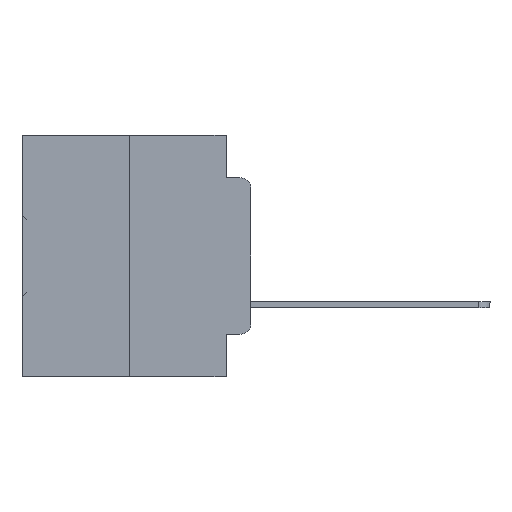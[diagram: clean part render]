
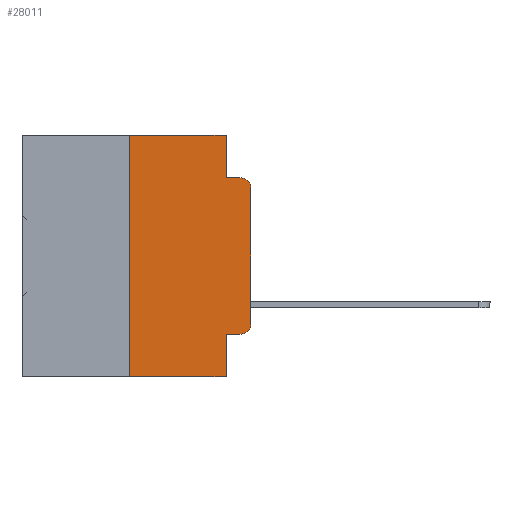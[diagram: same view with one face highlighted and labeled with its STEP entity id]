
A CAD part, left-side view. The second image highlights one B-rep face of the part: STEP entity #28011.
In plain terms, the highlighted planar face has unit normal (-1, 0, 0).
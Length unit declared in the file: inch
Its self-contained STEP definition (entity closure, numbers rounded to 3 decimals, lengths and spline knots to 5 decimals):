
#132 = VECTOR ( 'NONE', #17578, 39.37008 ) ;
#2353 = VERTEX_POINT ( 'NONE', #35481 ) ;
#2831 = DIRECTION ( 'NONE',  ( 0., 0., -1. ) ) ;
#4867 = VERTEX_POINT ( 'NONE', #15763 ) ;
#5420 = ORIENTED_EDGE ( 'NONE', *, *, #31383, .T. ) ;
#5552 = EDGE_CURVE ( 'NONE', #30710, #17020, #28559, .T. ) ;
#5701 = EDGE_CURVE ( 'NONE', #6579, #4867, #35004, .T. ) ;
#6166 = VECTOR ( 'NONE', #27151, 39.37008 ) ;
#6307 = VERTEX_POINT ( 'NONE', #22232 ) ;
#6451 = VECTOR ( 'NONE', #31825, 39.37008 ) ;
#6579 = VERTEX_POINT ( 'NONE', #26441 ) ;
#6955 = CARTESIAN_POINT ( 'NONE',  ( 0., 0.051, 0. ) ) ;
#7369 = ORIENTED_EDGE ( 'NONE', *, *, #24601, .F. ) ;
#7588 = VECTOR ( 'NONE', #8814, 39.37008 ) ;
#7615 = VERTEX_POINT ( 'NONE', #15172 ) ;
#8107 = CIRCLE ( 'NONE', #23387, 0.02 ) ;
#8814 = DIRECTION ( 'NONE',  ( 0., 0., 1. ) ) ;
#8893 = ORIENTED_EDGE ( 'NONE', *, *, #24710, .T. ) ;
#9020 = DIRECTION ( 'NONE',  ( 0., -1., 0. ) ) ;
#9354 = LINE ( 'NONE', #6955, #6451 ) ;
#9924 = ORIENTED_EDGE ( 'NONE', *, *, #27396, .F. ) ;
#10054 = VERTEX_POINT ( 'NONE', #34585 ) ;
#11813 = ORIENTED_EDGE ( 'NONE', *, *, #5701, .T. ) ;
#12061 = LINE ( 'NONE', #31401, #132 ) ;
#12445 = EDGE_CURVE ( 'NONE', #6579, #7615, #9354, .T. ) ;
#15172 = CARTESIAN_POINT ( 'NONE',  ( 0., 0.051, -0.5 ) ) ;
#15763 = CARTESIAN_POINT ( 'NONE',  ( 0., 0.02, -0.4115 ) ) ;
#16089 = LINE ( 'NONE', #27339, #6166 ) ;
#16677 = VERTEX_POINT ( 'NONE', #23759 ) ;
#16905 = CARTESIAN_POINT ( 'NONE',  ( 0., 0., -0.3915 ) ) ;
#16954 = DIRECTION ( 'NONE',  ( 0., 0., -1. ) ) ;
#17020 = VERTEX_POINT ( 'NONE', #25204 ) ;
#17578 = DIRECTION ( 'NONE',  ( 0., 0., -1. ) ) ;
#17596 = CARTESIAN_POINT ( 'NONE',  ( 0., 0.473, 0. ) ) ;
#17858 = DIRECTION ( 'NONE',  ( 1., 0., 0. ) ) ;
#18437 = ORIENTED_EDGE ( 'NONE', *, *, #36356, .F. ) ;
#18599 = ORIENTED_EDGE ( 'NONE', *, *, #12445, .F. ) ;
#19317 = EDGE_LOOP ( 'NONE', ( #5420, #32212, #31492, #18437, #9924, #7369, #24969, #18599, #11813, #8893 ) ) ;
#19327 = AXIS2_PLACEMENT_3D ( 'NONE', #20994, #17858, #29653 ) ;
#19458 = VERTEX_POINT ( 'NONE', #16905 ) ;
#20444 = VECTOR ( 'NONE', #31789, 39.37008 ) ;
#20994 = CARTESIAN_POINT ( 'NONE',  ( 0., 0.473, 0. ) ) ;
#22232 = CARTESIAN_POINT ( 'NONE',  ( 0., 0., -0.1085 ) ) ;
#23070 = DIRECTION ( 'NONE',  ( -1., 0., 0. ) ) ;
#23387 = AXIS2_PLACEMENT_3D ( 'NONE', #28196, #31681, #16954 ) ;
#23759 = CARTESIAN_POINT ( 'NONE',  ( 0., 0.051, 0. ) ) ;
#24179 = LINE ( 'NONE', #35405, #32360 ) ;
#24601 = EDGE_CURVE ( 'NONE', #2353, #10054, #16089, .T. ) ;
#24710 = EDGE_CURVE ( 'NONE', #4867, #19458, #26739, .T. ) ;
#24969 = ORIENTED_EDGE ( 'NONE', *, *, #34084, .T. ) ;
#24986 = VECTOR ( 'NONE', #9020, 39.37008 ) ;
#25204 = CARTESIAN_POINT ( 'NONE',  ( 0., 0.02, -0.0885 ) ) ;
#26441 = CARTESIAN_POINT ( 'NONE',  ( 0., 0.051, -0.4115 ) ) ;
#26739 = CIRCLE ( 'NONE', #29680, 0.02 ) ;
#27151 = DIRECTION ( 'NONE',  ( 0., 0., 1. ) ) ;
#27339 = CARTESIAN_POINT ( 'NONE',  ( 0., 0.25, 0. ) ) ;
#27396 = EDGE_CURVE ( 'NONE', #10054, #16677, #34922, .T. ) ;
#27898 = EDGE_CURVE ( 'NONE', #6307, #17020, #8107, .T. ) ;
#28011 = ADVANCED_FACE ( 'NONE', ( #29118 ), #35173, .F. ) ;
#28196 = CARTESIAN_POINT ( 'NONE',  ( 0., 0.02, -0.1085 ) ) ;
#28538 = LINE ( 'NONE', #34056, #7588 ) ;
#28559 = LINE ( 'NONE', #34450, #24986 ) ;
#29118 = FACE_OUTER_BOUND ( 'NONE', #19317, .T. ) ;
#29653 = DIRECTION ( 'NONE',  ( 0., 0., -1. ) ) ;
#29680 = AXIS2_PLACEMENT_3D ( 'NONE', #34492, #23070, #2831 ) ;
#29869 = DIRECTION ( 'NONE',  ( 0., -1., 0. ) ) ;
#30710 = VERTEX_POINT ( 'NONE', #35792 ) ;
#31383 = EDGE_CURVE ( 'NONE', #19458, #6307, #28538, .T. ) ;
#31401 = CARTESIAN_POINT ( 'NONE',  ( 0., 0.051, 0. ) ) ;
#31432 = VECTOR ( 'NONE', #35540, 39.37008 ) ;
#31492 = ORIENTED_EDGE ( 'NONE', *, *, #5552, .F. ) ;
#31681 = DIRECTION ( 'NONE',  ( -1., 0., 0. ) ) ;
#31789 = DIRECTION ( 'NONE',  ( 0., -1., 0. ) ) ;
#31825 = DIRECTION ( 'NONE',  ( 0., 0., -1. ) ) ;
#32212 = ORIENTED_EDGE ( 'NONE', *, *, #27898, .T. ) ;
#32360 = VECTOR ( 'NONE', #29869, 39.37008 ) ;
#34056 = CARTESIAN_POINT ( 'NONE',  ( 0., 0., 0. ) ) ;
#34084 = EDGE_CURVE ( 'NONE', #2353, #7615, #24179, .T. ) ;
#34450 = CARTESIAN_POINT ( 'NONE',  ( 0., 0.051, -0.0885 ) ) ;
#34492 = CARTESIAN_POINT ( 'NONE',  ( 0., 0.02, -0.3915 ) ) ;
#34585 = CARTESIAN_POINT ( 'NONE',  ( 0., 0.25, 0. ) ) ;
#34922 = LINE ( 'NONE', #17596, #20444 ) ;
#35004 = LINE ( 'NONE', #35167, #31432 ) ;
#35167 = CARTESIAN_POINT ( 'NONE',  ( 0., 0.051, -0.4115 ) ) ;
#35173 = PLANE ( 'NONE',  #19327 ) ;
#35405 = CARTESIAN_POINT ( 'NONE',  ( 0., 0.473, -0.5 ) ) ;
#35481 = CARTESIAN_POINT ( 'NONE',  ( 0., 0.25, -0.5 ) ) ;
#35540 = DIRECTION ( 'NONE',  ( 0., -1., 0. ) ) ;
#35792 = CARTESIAN_POINT ( 'NONE',  ( 0., 0.051, -0.0885 ) ) ;
#36356 = EDGE_CURVE ( 'NONE', #16677, #30710, #12061, .T. ) ;
